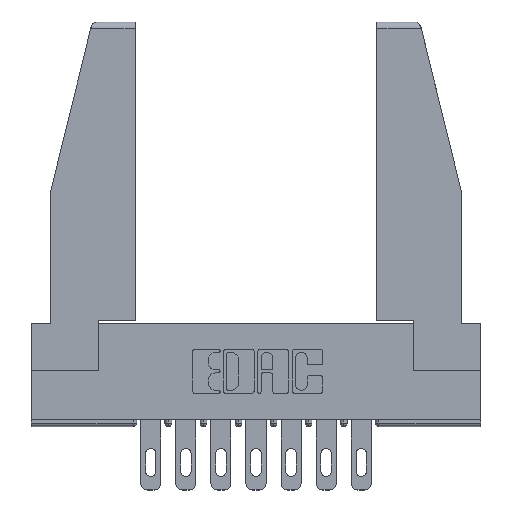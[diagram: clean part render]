
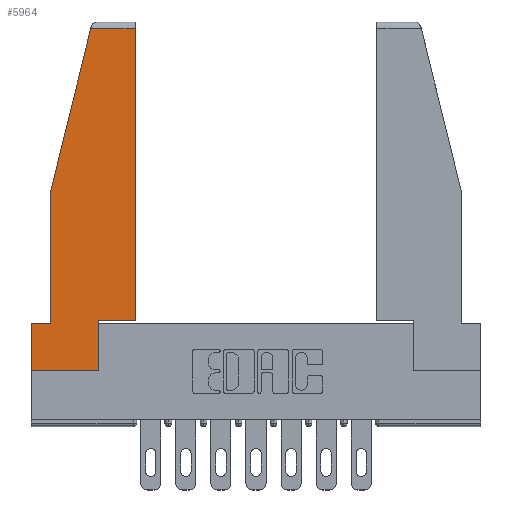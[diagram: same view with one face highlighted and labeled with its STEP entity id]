
A CAD part, top view. The second image highlights one B-rep face of the part: STEP entity #5964.
In plain terms, the highlighted planar face has unit normal (0, 0, 1).
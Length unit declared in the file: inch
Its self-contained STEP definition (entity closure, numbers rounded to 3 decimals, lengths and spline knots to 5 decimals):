
#254 = VERTEX_POINT ( 'NONE', #2282 ) ;
#691 = EDGE_CURVE ( 'NONE', #7648, #8801, #3375, .T. ) ;
#752 = LINE ( 'NONE', #2682, #12191 ) ;
#834 = PLANE ( 'NONE',  #5026 ) ;
#1006 = ORIENTED_EDGE ( 'NONE', *, *, #6146, .T. ) ;
#1108 = EDGE_LOOP ( 'NONE', ( #6995, #6949, #13885, #13547, #12288, #1006, #1545, #5921, #2508 ) ) ;
#1545 = ORIENTED_EDGE ( 'NONE', *, *, #8707, .T. ) ;
#1556 = EDGE_CURVE ( 'NONE', #10656, #10054, #4894, .T. ) ;
#1713 = DIRECTION ( 'NONE',  ( -1., 0., 0. ) ) ;
#2094 = DIRECTION ( 'NONE',  ( 0., 1., 0. ) ) ;
#2282 = CARTESIAN_POINT ( 'NONE',  ( 0.297, 0.223, 0. ) ) ;
#2338 = VECTOR ( 'NONE', #8989, 39.37008 ) ;
#2508 = ORIENTED_EDGE ( 'NONE', *, *, #13207, .T. ) ;
#2682 = CARTESIAN_POINT ( 'NONE',  ( 0.271, 1.55, 0. ) ) ;
#2892 = EDGE_CURVE ( 'NONE', #5055, #10656, #12004, .T. ) ;
#2896 = EDGE_CURVE ( 'NONE', #4659, #254, #14045, .T. ) ;
#3351 = LINE ( 'NONE', #7767, #7528 ) ;
#3375 = LINE ( 'NONE', #7680, #2338 ) ;
#3384 = CARTESIAN_POINT ( 'NONE',  ( 0., 0.21, 0. ) ) ;
#3431 = CARTESIAN_POINT ( 'NONE',  ( 0.461, 1.52, 0. ) ) ;
#4194 = VERTEX_POINT ( 'NONE', #10339 ) ;
#4277 = DIRECTION ( 'NONE',  ( 0., -1., 0. ) ) ;
#4571 = CARTESIAN_POINT ( 'NONE',  ( 0.297, 0.223, 0. ) ) ;
#4659 = VERTEX_POINT ( 'NONE', #11051 ) ;
#4731 = LINE ( 'NONE', #10589, #13408 ) ;
#4835 = LINE ( 'NONE', #4571, #5355 ) ;
#4867 = CARTESIAN_POINT ( 'NONE',  ( 0., 0., 0. ) ) ;
#4894 = LINE ( 'NONE', #10513, #9416 ) ;
#4904 = DIRECTION ( 'NONE',  ( -0.239, -0.971, 0. ) ) ;
#4998 = CARTESIAN_POINT ( 'NONE',  ( 0.461, 0.223, 0. ) ) ;
#5026 = AXIS2_PLACEMENT_3D ( 'NONE', #10805, #9666, #8669 ) ;
#5055 = VERTEX_POINT ( 'NONE', #4998 ) ;
#5355 = VECTOR ( 'NONE', #12365, 39.37008 ) ;
#5521 = VECTOR ( 'NONE', #9774, 39.37008 ) ;
#5609 = FACE_OUTER_BOUND ( 'NONE', #1108, .T. ) ;
#5921 = ORIENTED_EDGE ( 'NONE', *, *, #2896, .T. ) ;
#5964 = ADVANCED_FACE ( 'NONE', ( #5609 ), #834, .T. ) ;
#6045 = LINE ( 'NONE', #7525, #5521 ) ;
#6146 = EDGE_CURVE ( 'NONE', #8801, #8217, #4731, .T. ) ;
#6199 = EDGE_CURVE ( 'NONE', #4194, #7648, #3351, .T. ) ;
#6949 = ORIENTED_EDGE ( 'NONE', *, *, #1556, .T. ) ;
#6995 = ORIENTED_EDGE ( 'NONE', *, *, #2892, .T. ) ;
#7359 = EDGE_CURVE ( 'NONE', #10054, #4194, #752, .T. ) ;
#7525 = CARTESIAN_POINT ( 'NONE',  ( 0., 0., 0. ) ) ;
#7528 = VECTOR ( 'NONE', #9980, 39.37008 ) ;
#7648 = VERTEX_POINT ( 'NONE', #9238 ) ;
#7680 = CARTESIAN_POINT ( 'NONE',  ( 0., 0.21, 0. ) ) ;
#7767 = CARTESIAN_POINT ( 'NONE',  ( 0.086, 0.8, 0. ) ) ;
#7806 = DIRECTION ( 'NONE',  ( 0., 1., 0. ) ) ;
#8217 = VERTEX_POINT ( 'NONE', #4867 ) ;
#8669 = DIRECTION ( 'NONE',  ( 1., 0., 0. ) ) ;
#8707 = EDGE_CURVE ( 'NONE', #8217, #4659, #6045, .T. ) ;
#8801 = VERTEX_POINT ( 'NONE', #3384 ) ;
#8989 = DIRECTION ( 'NONE',  ( -1., 0., 0. ) ) ;
#9238 = CARTESIAN_POINT ( 'NONE',  ( 0.086, 0.21, 0. ) ) ;
#9416 = VECTOR ( 'NONE', #1713, 39.37008 ) ;
#9666 = DIRECTION ( 'NONE',  ( 0., 0., 1. ) ) ;
#9774 = DIRECTION ( 'NONE',  ( 1., 0., 0. ) ) ;
#9966 = CARTESIAN_POINT ( 'NONE',  ( 0.297, 0., 0. ) ) ;
#9980 = DIRECTION ( 'NONE',  ( 0., -1., 0. ) ) ;
#10054 = VERTEX_POINT ( 'NONE', #12754 ) ;
#10339 = CARTESIAN_POINT ( 'NONE',  ( 0.086, 0.8, 0. ) ) ;
#10513 = CARTESIAN_POINT ( 'NONE',  ( 0., 1.52, 0. ) ) ;
#10589 = CARTESIAN_POINT ( 'NONE',  ( 0., 0.21, 0. ) ) ;
#10656 = VERTEX_POINT ( 'NONE', #3431 ) ;
#10805 = CARTESIAN_POINT ( 'NONE',  ( 0., 0., 0. ) ) ;
#11051 = CARTESIAN_POINT ( 'NONE',  ( 0.297, 0., 0. ) ) ;
#11148 = VECTOR ( 'NONE', #2094, 39.37008 ) ;
#12004 = LINE ( 'NONE', #14269, #12345 ) ;
#12191 = VECTOR ( 'NONE', #4904, 39.37008 ) ;
#12288 = ORIENTED_EDGE ( 'NONE', *, *, #691, .T. ) ;
#12345 = VECTOR ( 'NONE', #7806, 39.37008 ) ;
#12365 = DIRECTION ( 'NONE',  ( 1., 0., 0. ) ) ;
#12754 = CARTESIAN_POINT ( 'NONE',  ( 0.2636, 1.52, 0. ) ) ;
#13207 = EDGE_CURVE ( 'NONE', #254, #5055, #4835, .T. ) ;
#13408 = VECTOR ( 'NONE', #4277, 39.37008 ) ;
#13547 = ORIENTED_EDGE ( 'NONE', *, *, #6199, .T. ) ;
#13885 = ORIENTED_EDGE ( 'NONE', *, *, #7359, .T. ) ;
#14045 = LINE ( 'NONE', #9966, #11148 ) ;
#14269 = CARTESIAN_POINT ( 'NONE',  ( 0.461, 0.223, 0. ) ) ;
